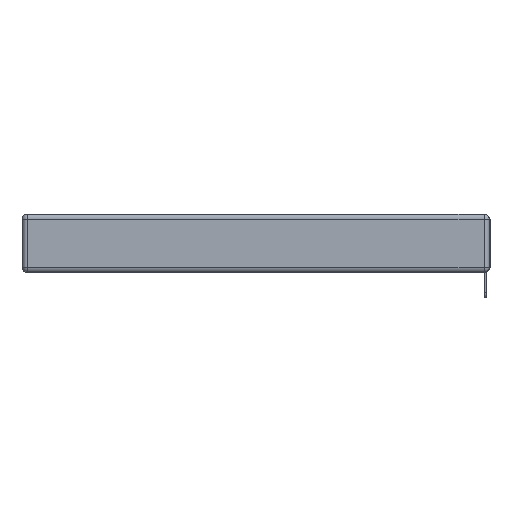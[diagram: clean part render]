
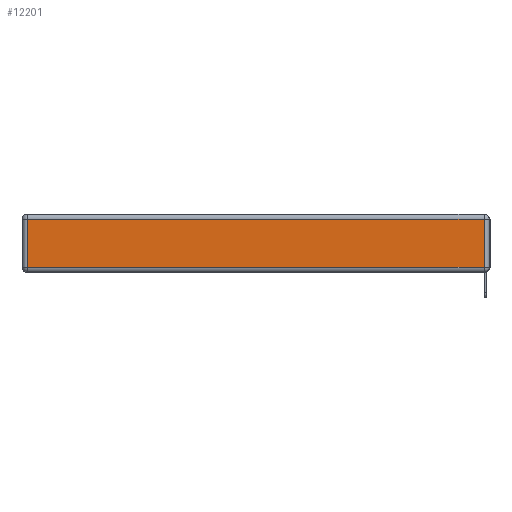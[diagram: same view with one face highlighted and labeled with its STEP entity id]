
A CAD part, left-side view. The second image highlights one B-rep face of the part: STEP entity #12201.
In plain terms, the highlighted planar face has unit normal (-1, 0, 0).
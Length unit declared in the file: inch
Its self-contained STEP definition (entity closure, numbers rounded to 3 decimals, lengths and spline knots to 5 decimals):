
#217 = VECTOR ( 'NONE', #13611, 39.37008 ) ;
#262 = CARTESIAN_POINT ( 'NONE',  ( 0., 0.03, -0.343 ) ) ;
#317 = CARTESIAN_POINT ( 'NONE',  ( 0., 0., -0.343 ) ) ;
#426 = EDGE_CURVE ( 'NONE', #20681, #10132, #10323, .T. ) ;
#1914 = VECTOR ( 'NONE', #6913, 39.37008 ) ;
#2187 = CARTESIAN_POINT ( 'NONE',  ( 0., 0., -0.313 ) ) ;
#2298 = ORIENTED_EDGE ( 'NONE', *, *, #21016, .T. ) ;
#3474 = LINE ( 'NONE', #262, #1914 ) ;
#5031 = ORIENTED_EDGE ( 'NONE', *, *, #9403, .T. ) ;
#5658 = VERTEX_POINT ( 'NONE', #17881 ) ;
#6377 = FACE_OUTER_BOUND ( 'NONE', #19418, .T. ) ;
#6913 = DIRECTION ( 'NONE',  ( 0., 0., 1. ) ) ;
#6961 = PLANE ( 'NONE',  #16809 ) ;
#8089 = CARTESIAN_POINT ( 'NONE',  ( 0., 2.75, -0.03 ) ) ;
#8223 = ORIENTED_EDGE ( 'NONE', *, *, #16236, .T. ) ;
#8348 = DIRECTION ( 'NONE',  ( 0., 0., 1. ) ) ;
#9403 = EDGE_CURVE ( 'NONE', #19712, #20681, #15913, .T. ) ;
#9944 = CARTESIAN_POINT ( 'NONE',  ( 0., 2.72, -0.03 ) ) ;
#10132 = VERTEX_POINT ( 'NONE', #15730 ) ;
#10323 = LINE ( 'NONE', #2187, #217 ) ;
#12201 = ADVANCED_FACE ( 'NONE', ( #6377 ), #6961, .T. ) ;
#13221 = DIRECTION ( 'NONE',  ( 0., 1., 0. ) ) ;
#13522 = VECTOR ( 'NONE', #13221, 39.37008 ) ;
#13611 = DIRECTION ( 'NONE',  ( 0., -1., 0. ) ) ;
#15221 = CARTESIAN_POINT ( 'NONE',  ( 0., 2.72, -0.343 ) ) ;
#15730 = CARTESIAN_POINT ( 'NONE',  ( 0., 0.03, -0.313 ) ) ;
#15913 = LINE ( 'NONE', #15221, #19252 ) ;
#16236 = EDGE_CURVE ( 'NONE', #5658, #19712, #16880, .T. ) ;
#16809 = AXIS2_PLACEMENT_3D ( 'NONE', #317, #18394, #8348 ) ;
#16880 = LINE ( 'NONE', #8089, #13522 ) ;
#17881 = CARTESIAN_POINT ( 'NONE',  ( 0., 0.03, -0.03 ) ) ;
#18394 = DIRECTION ( 'NONE',  ( -1., 0., 0. ) ) ;
#19075 = ORIENTED_EDGE ( 'NONE', *, *, #426, .T. ) ;
#19252 = VECTOR ( 'NONE', #20582, 39.37008 ) ;
#19403 = CARTESIAN_POINT ( 'NONE',  ( 0., 2.72, -0.313 ) ) ;
#19418 = EDGE_LOOP ( 'NONE', ( #19075, #2298, #8223, #5031 ) ) ;
#19712 = VERTEX_POINT ( 'NONE', #9944 ) ;
#20582 = DIRECTION ( 'NONE',  ( 0., 0., -1. ) ) ;
#20681 = VERTEX_POINT ( 'NONE', #19403 ) ;
#21016 = EDGE_CURVE ( 'NONE', #10132, #5658, #3474, .T. ) ;
